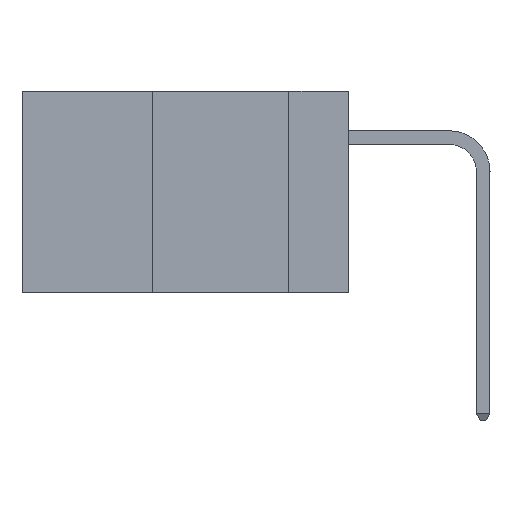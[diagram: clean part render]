
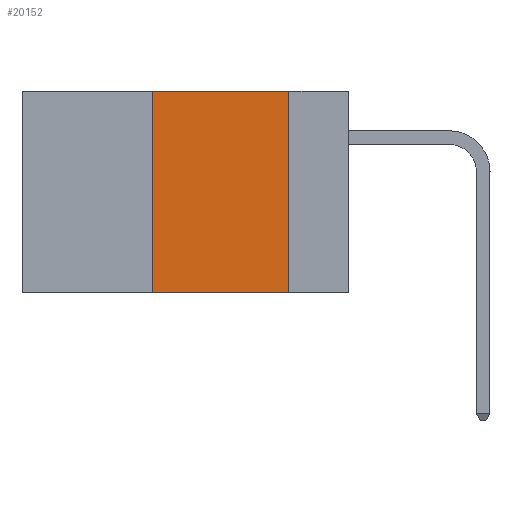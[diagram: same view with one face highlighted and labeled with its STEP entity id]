
A CAD part, left-side view. The second image highlights one B-rep face of the part: STEP entity #20152.
In plain terms, the highlighted planar face has unit normal (-1, 0, 0).
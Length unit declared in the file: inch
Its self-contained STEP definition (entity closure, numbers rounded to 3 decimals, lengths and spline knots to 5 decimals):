
#61 = VERTEX_POINT ( 'NONE', #24974 ) ;
#697 = ORIENTED_EDGE ( 'NONE', *, *, #22681, .F. ) ;
#1882 = PLANE ( 'NONE',  #32144 ) ;
#2462 = VECTOR ( 'NONE', #23229, 39.37008 ) ;
#2762 = VERTEX_POINT ( 'NONE', #5813 ) ;
#4272 = CARTESIAN_POINT ( 'NONE',  ( 0., 0.6, -0.37 ) ) ;
#5813 = CARTESIAN_POINT ( 'NONE',  ( 0., 0.11, 0. ) ) ;
#9503 = FACE_OUTER_BOUND ( 'NONE', #17327, .T. ) ;
#11796 = ORIENTED_EDGE ( 'NONE', *, *, #16383, .T. ) ;
#11955 = ORIENTED_EDGE ( 'NONE', *, *, #23550, .F. ) ;
#14107 = VECTOR ( 'NONE', #31822, 39.37008 ) ;
#14653 = DIRECTION ( 'NONE',  ( 1., 0., 0. ) ) ;
#14870 = CARTESIAN_POINT ( 'NONE',  ( 0., 0.36, -0.37 ) ) ;
#15058 = VECTOR ( 'NONE', #25910, 39.37008 ) ;
#16383 = EDGE_CURVE ( 'NONE', #28849, #29591, #19918, .T. ) ;
#17327 = EDGE_LOOP ( 'NONE', ( #697, #23737, #11955, #11796 ) ) ;
#19658 = CARTESIAN_POINT ( 'NONE',  ( 0., 0.6, 0. ) ) ;
#19918 = LINE ( 'NONE', #4272, #32471 ) ;
#20152 = ADVANCED_FACE ( 'NONE', ( #9503 ), #1882, .F. ) ;
#21479 = CARTESIAN_POINT ( 'NONE',  ( 0., 0.11, -0.37 ) ) ;
#22681 = EDGE_CURVE ( 'NONE', #2762, #29591, #29491, .T. ) ;
#23229 = DIRECTION ( 'NONE',  ( 0., 0., 1. ) ) ;
#23550 = EDGE_CURVE ( 'NONE', #28849, #61, #30537, .T. ) ;
#23737 = ORIENTED_EDGE ( 'NONE', *, *, #30431, .F. ) ;
#24835 = DIRECTION ( 'NONE',  ( 0., 0., -1. ) ) ;
#24974 = CARTESIAN_POINT ( 'NONE',  ( 0., 0.36, 0. ) ) ;
#25068 = DIRECTION ( 'NONE',  ( 0., -1., 0. ) ) ;
#25884 = CARTESIAN_POINT ( 'NONE',  ( 0., 0.36, 0. ) ) ;
#25910 = DIRECTION ( 'NONE',  ( 0., -1., 0. ) ) ;
#26499 = CARTESIAN_POINT ( 'NONE',  ( 0., 0.11, 0. ) ) ;
#28401 = LINE ( 'NONE', #28568, #15058 ) ;
#28568 = CARTESIAN_POINT ( 'NONE',  ( 0., 0.6, 0. ) ) ;
#28849 = VERTEX_POINT ( 'NONE', #14870 ) ;
#29491 = LINE ( 'NONE', #26499, #14107 ) ;
#29591 = VERTEX_POINT ( 'NONE', #21479 ) ;
#30431 = EDGE_CURVE ( 'NONE', #61, #2762, #28401, .T. ) ;
#30537 = LINE ( 'NONE', #25884, #2462 ) ;
#31822 = DIRECTION ( 'NONE',  ( 0., 0., -1. ) ) ;
#32144 = AXIS2_PLACEMENT_3D ( 'NONE', #19658, #14653, #24835 ) ;
#32471 = VECTOR ( 'NONE', #25068, 39.37008 ) ;
